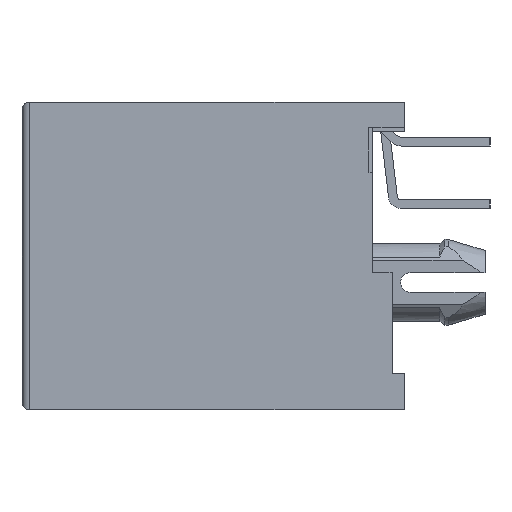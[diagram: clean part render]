
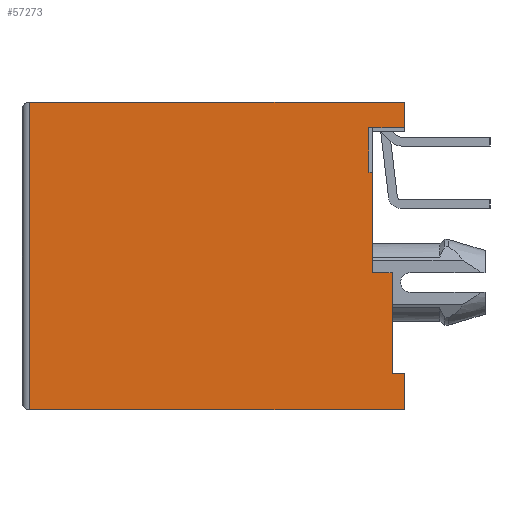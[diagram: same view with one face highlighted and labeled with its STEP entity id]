
A CAD part, left-side view. The second image highlights one B-rep face of the part: STEP entity #57273.
In plain terms, the highlighted planar face has unit normal (-1, 0, 0).
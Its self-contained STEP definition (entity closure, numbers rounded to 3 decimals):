
#90 = VERTEX_POINT ( 'NONE', #20249 ) ;
#850 = CARTESIAN_POINT ( 'NONE',  ( -31.5, 7.5, -6.25 ) ) ;
#960 = CARTESIAN_POINT ( 'NONE',  ( -31.5, -6.35, 3.45 ) ) ;
#2582 = B_SPLINE_CURVE_WITH_KNOTS ( 'NONE', 3,
 ( #44050, #44380, #33731, #24061 ),
 .UNSPECIFIED., .F., .F.,
 ( 4, 4 ),
 ( 0., 1. ),
 .UNSPECIFIED. ) ;
#2939 = CARTESIAN_POINT ( 'NONE',  ( -31.5, -6.5, -0.65 ) ) ;
#3439 = ORIENTED_EDGE ( 'NONE', *, *, #29141, .F. ) ;
#3463 = CARTESIAN_POINT ( 'NONE',  ( -31.5, 7.5, 6.3 ) ) ;
#3747 = VERTEX_POINT ( 'NONE', #20077 ) ;
#3774 = AXIS2_PLACEMENT_3D ( 'NONE', #20821, #52836, #21491 ) ;
#5013 = EDGE_CURVE ( 'NONE', #64334, #65012, #68112, .T. ) ;
#5242 = EDGE_CURVE ( 'NONE', #90, #29605, #54925, .T. ) ;
#6452 = ORIENTED_EDGE ( 'NONE', *, *, #45047, .T. ) ;
#7068 = CARTESIAN_POINT ( 'NONE',  ( -31.5, -6.4, 3.45 ) ) ;
#7372 = CARTESIAN_POINT ( 'NONE',  ( -31.5, -6.35, 4.05 ) ) ;
#7471 = ORIENTED_EDGE ( 'NONE', *, *, #17818, .F. ) ;
#8960 = EDGE_LOOP ( 'NONE', ( #3439, #19261, #19707, #49055, #7471, #54894, #60563, #27316, #25006, #18785, #6452, #39620 ) ) ;
#9003 = CARTESIAN_POINT ( 'NONE',  ( -31.5, -7.8, -4.75 ) ) ;
#10124 = CARTESIAN_POINT ( 'NONE',  ( -31.5, -7.8, -6.25 ) ) ;
#10260 = CARTESIAN_POINT ( 'NONE',  ( -31.5, -7.3, -4.75 ) ) ;
#12925 = CARTESIAN_POINT ( 'NONE',  ( -31.5, -6.5, 3.45 ) ) ;
#13268 = CARTESIAN_POINT ( 'NONE',  ( -31.5, -6.5, 0.717 ) ) ;
#13964 = CARTESIAN_POINT ( 'NONE',  ( -31.5, -7.3, -0.65 ) ) ;
#14874 = CARTESIAN_POINT ( 'NONE',  ( -31.5, -6.5, 3.45 ) ) ;
#15070 = CARTESIAN_POINT ( 'NONE',  ( -31.5, 7.5, 2.117 ) ) ;
#15706 = CARTESIAN_POINT ( 'NONE',  ( -31.5, -6.35, 3.45 ) ) ;
#17818 = EDGE_CURVE ( 'NONE', #65012, #59400, #22979, .T. ) ;
#17921 = CARTESIAN_POINT ( 'NONE',  ( -31.5, -7.8, 5.25 ) ) ;
#18050 = B_SPLINE_CURVE_WITH_KNOTS ( 'NONE', 3,
 ( #13964, #62108, #46281, #51781 ),
 .UNSPECIFIED., .F., .F.,
 ( 4, 4 ),
 ( 0., 1. ),
 .UNSPECIFIED. ) ;
#18785 = ORIENTED_EDGE ( 'NONE', *, *, #41041, .T. ) ;
#19261 = ORIENTED_EDGE ( 'NONE', *, *, #57218, .F. ) ;
#19707 = ORIENTED_EDGE ( 'NONE', *, *, #43804, .F. ) ;
#19828 = CARTESIAN_POINT ( 'NONE',  ( -31.5, -7.8, -4.75 ) ) ;
#20077 = CARTESIAN_POINT ( 'NONE',  ( -31.5, 7.5, -6.25 ) ) ;
#20249 = CARTESIAN_POINT ( 'NONE',  ( -31.5, -7.8, 6.3 ) ) ;
#20482 = FACE_OUTER_BOUND ( 'NONE', #8960, .T. ) ;
#20821 = CARTESIAN_POINT ( 'NONE',  ( -31.5, 7.806, -6.501 ) ) ;
#20946 = CARTESIAN_POINT ( 'NONE',  ( -31.5, -7.8, 5.25 ) ) ;
#21491 = DIRECTION ( 'NONE',  ( 0., 0., 1. ) ) ;
#22158 = CARTESIAN_POINT ( 'NONE',  ( -31.5, -7.3, -0.65 ) ) ;
#22955 = CARTESIAN_POINT ( 'NONE',  ( -31.5, -6.35, 5.25 ) ) ;
#22979 = B_SPLINE_CURVE_WITH_KNOTS ( 'NONE', 3,
 ( #60408, #50068, #13268, #2939 ),
 .UNSPECIFIED., .F., .F.,
 ( 4, 4 ),
 ( 0., 1. ),
 .UNSPECIFIED. ) ;
#23526 = CARTESIAN_POINT ( 'NONE',  ( -31.5, -6.35, 4.65 ) ) ;
#24061 = CARTESIAN_POINT ( 'NONE',  ( -31.5, -7.3, -0.65 ) ) ;
#24262 = CARTESIAN_POINT ( 'NONE',  ( -31.5, 7.5, 6.3 ) ) ;
#24264 = EDGE_CURVE ( 'NONE', #33237, #64334, #55528, .T. ) ;
#24293 = CARTESIAN_POINT ( 'NONE',  ( -31.5, -7.8, -4.75 ) ) ;
#24596 = CARTESIAN_POINT ( 'NONE',  ( -31.5, -2.7, 6.3 ) ) ;
#25006 = ORIENTED_EDGE ( 'NONE', *, *, #5242, .F. ) ;
#27300 = B_SPLINE_CURVE_WITH_KNOTS ( 'NONE', 3,
 ( #9003, #60979, #40330, #29664 ),
 .UNSPECIFIED., .F., .F.,
 ( 4, 4 ),
 ( 0., 1. ),
 .UNSPECIFIED. ) ;
#27316 = ORIENTED_EDGE ( 'NONE', *, *, #39235, .F. ) ;
#28235 = CARTESIAN_POINT ( 'NONE',  ( -31.5, -7.8, 5.95 ) ) ;
#28786 = B_SPLINE_CURVE_WITH_KNOTS ( 'NONE', 3,
 ( #66648, #29790, #34642, #24293 ),
 .UNSPECIFIED., .F., .F.,
 ( 4, 4 ),
 ( 0., 1. ),
 .UNSPECIFIED. ) ;
#29063 = CARTESIAN_POINT ( 'NONE',  ( -31.5, -6.45, 3.45 ) ) ;
#29141 = EDGE_CURVE ( 'NONE', #51658, #56260, #27300, .T. ) ;
#29605 = VERTEX_POINT ( 'NONE', #20946 ) ;
#29664 = CARTESIAN_POINT ( 'NONE',  ( -31.5, -7.8, -6.25 ) ) ;
#29790 = CARTESIAN_POINT ( 'NONE',  ( -31.5, -7.467, -4.75 ) ) ;
#30801 = PLANE ( 'NONE',  #3774 ) ;
#31117 = CARTESIAN_POINT ( 'NONE',  ( -31.5, 2.4, -6.25 ) ) ;
#33237 = VERTEX_POINT ( 'NONE', #22955 ) ;
#33731 = CARTESIAN_POINT ( 'NONE',  ( -31.5, -7.033, -0.65 ) ) ;
#34642 = CARTESIAN_POINT ( 'NONE',  ( -31.5, -7.633, -4.75 ) ) ;
#35392 = CARTESIAN_POINT ( 'NONE',  ( -31.5, 7.5, -6.25 ) ) ;
#36716 = EDGE_CURVE ( 'NONE', #56260, #3747, #62236, .T. ) ;
#39189 = B_SPLINE_CURVE_WITH_KNOTS ( 'NONE', 3,
 ( #65249, #24596, #65600, #24262 ),
 .UNSPECIFIED., .F., .F.,
 ( 4, 4 ),
 ( 0., 1. ),
 .UNSPECIFIED. ) ;
#39235 = EDGE_CURVE ( 'NONE', #29605, #33237, #61555, .T. ) ;
#39246 = CARTESIAN_POINT ( 'NONE',  ( -31.5, -6.833, 5.25 ) ) ;
#39620 = ORIENTED_EDGE ( 'NONE', *, *, #36716, .F. ) ;
#40330 = CARTESIAN_POINT ( 'NONE',  ( -31.5, -7.8, -5.75 ) ) ;
#40871 = CARTESIAN_POINT ( 'NONE',  ( -31.5, 7.5, -2.067 ) ) ;
#41041 = EDGE_CURVE ( 'NONE', #90, #65409, #39189, .T. ) ;
#43804 = EDGE_CURVE ( 'NONE', #45582, #62762, #18050, .T. ) ;
#44050 = CARTESIAN_POINT ( 'NONE',  ( -31.5, -6.5, -0.65 ) ) ;
#44380 = CARTESIAN_POINT ( 'NONE',  ( -31.5, -6.767, -0.65 ) ) ;
#45047 = EDGE_CURVE ( 'NONE', #65409, #3747, #50794, .T. ) ;
#45390 = CARTESIAN_POINT ( 'NONE',  ( -31.5, -6.35, 5.25 ) ) ;
#45582 = VERTEX_POINT ( 'NONE', #22158 ) ;
#46281 = CARTESIAN_POINT ( 'NONE',  ( -31.5, -7.3, -3.383 ) ) ;
#46704 = CARTESIAN_POINT ( 'NONE',  ( -31.5, 7.5, 6.3 ) ) ;
#48105 = CARTESIAN_POINT ( 'NONE',  ( -31.5, -6.35, 5.25 ) ) ;
#48897 = CARTESIAN_POINT ( 'NONE',  ( -31.5, -7.8, 6.3 ) ) ;
#49055 = ORIENTED_EDGE ( 'NONE', *, *, #52329, .F. ) ;
#50068 = CARTESIAN_POINT ( 'NONE',  ( -31.5, -6.5, 2.083 ) ) ;
#50794 = B_SPLINE_CURVE_WITH_KNOTS ( 'NONE', 3,
 ( #46704, #15070, #40871, #35392 ),
 .UNSPECIFIED., .F., .F.,
 ( 4, 4 ),
 ( 0., 1. ),
 .UNSPECIFIED. ) ;
#51658 = VERTEX_POINT ( 'NONE', #19828 ) ;
#51781 = CARTESIAN_POINT ( 'NONE',  ( -31.5, -7.3, -4.75 ) ) ;
#52329 = EDGE_CURVE ( 'NONE', #59400, #45582, #2582, .T. ) ;
#52836 = DIRECTION ( 'NONE',  ( 1., 0., 0. ) ) ;
#53499 = CARTESIAN_POINT ( 'NONE',  ( -31.5, -2.7, -6.25 ) ) ;
#54894 = ORIENTED_EDGE ( 'NONE', *, *, #5013, .F. ) ;
#54925 = B_SPLINE_CURVE_WITH_KNOTS ( 'NONE', 3,
 ( #48897, #28235, #64749, #17921 ),
 .UNSPECIFIED., .F., .F.,
 ( 4, 4 ),
 ( 0., 1. ),
 .UNSPECIFIED. ) ;
#55384 = CARTESIAN_POINT ( 'NONE',  ( -31.5, -7.317, 5.25 ) ) ;
#55470 = CARTESIAN_POINT ( 'NONE',  ( -31.5, -6.5, -0.65 ) ) ;
#55528 = B_SPLINE_CURVE_WITH_KNOTS ( 'NONE', 3,
 ( #48105, #23526, #7372, #960 ),
 .UNSPECIFIED., .F., .F.,
 ( 4, 4 ),
 ( 0., 1. ),
 .UNSPECIFIED. ) ;
#56260 = VERTEX_POINT ( 'NONE', #67648 ) ;
#57218 = EDGE_CURVE ( 'NONE', #62762, #51658, #28786, .T. ) ;
#57273 = ADVANCED_FACE ( 'NONE', ( #20482 ), #30801, .F. ) ;
#59400 = VERTEX_POINT ( 'NONE', #55470 ) ;
#59715 = CARTESIAN_POINT ( 'NONE',  ( -31.5, -6.35, 3.45 ) ) ;
#60408 = CARTESIAN_POINT ( 'NONE',  ( -31.5, -6.5, 3.45 ) ) ;
#60561 = CARTESIAN_POINT ( 'NONE',  ( -31.5, -7.8, 5.25 ) ) ;
#60563 = ORIENTED_EDGE ( 'NONE', *, *, #24264, .F. ) ;
#60979 = CARTESIAN_POINT ( 'NONE',  ( -31.5, -7.8, -5.25 ) ) ;
#61555 = B_SPLINE_CURVE_WITH_KNOTS ( 'NONE', 3,
 ( #60561, #55384, #39246, #45390 ),
 .UNSPECIFIED., .F., .F.,
 ( 4, 4 ),
 ( 0., 1. ),
 .UNSPECIFIED. ) ;
#62108 = CARTESIAN_POINT ( 'NONE',  ( -31.5, -7.3, -2.017 ) ) ;
#62236 = B_SPLINE_CURVE_WITH_KNOTS ( 'NONE', 3,
 ( #10124, #53499, #31117, #850 ),
 .UNSPECIFIED., .F., .F.,
 ( 4, 4 ),
 ( 0., 1. ),
 .UNSPECIFIED. ) ;
#62762 = VERTEX_POINT ( 'NONE', #10260 ) ;
#64334 = VERTEX_POINT ( 'NONE', #15706 ) ;
#64749 = CARTESIAN_POINT ( 'NONE',  ( -31.5, -7.8, 5.6 ) ) ;
#65012 = VERTEX_POINT ( 'NONE', #14874 ) ;
#65249 = CARTESIAN_POINT ( 'NONE',  ( -31.5, -7.8, 6.3 ) ) ;
#65409 = VERTEX_POINT ( 'NONE', #3463 ) ;
#65600 = CARTESIAN_POINT ( 'NONE',  ( -31.5, 2.4, 6.3 ) ) ;
#66648 = CARTESIAN_POINT ( 'NONE',  ( -31.5, -7.3, -4.75 ) ) ;
#67648 = CARTESIAN_POINT ( 'NONE',  ( -31.5, -7.8, -6.25 ) ) ;
#68112 = B_SPLINE_CURVE_WITH_KNOTS ( 'NONE', 3,
 ( #59715, #7068, #29063, #12925 ),
 .UNSPECIFIED., .F., .F.,
 ( 4, 4 ),
 ( 0., 1. ),
 .UNSPECIFIED. ) ;
